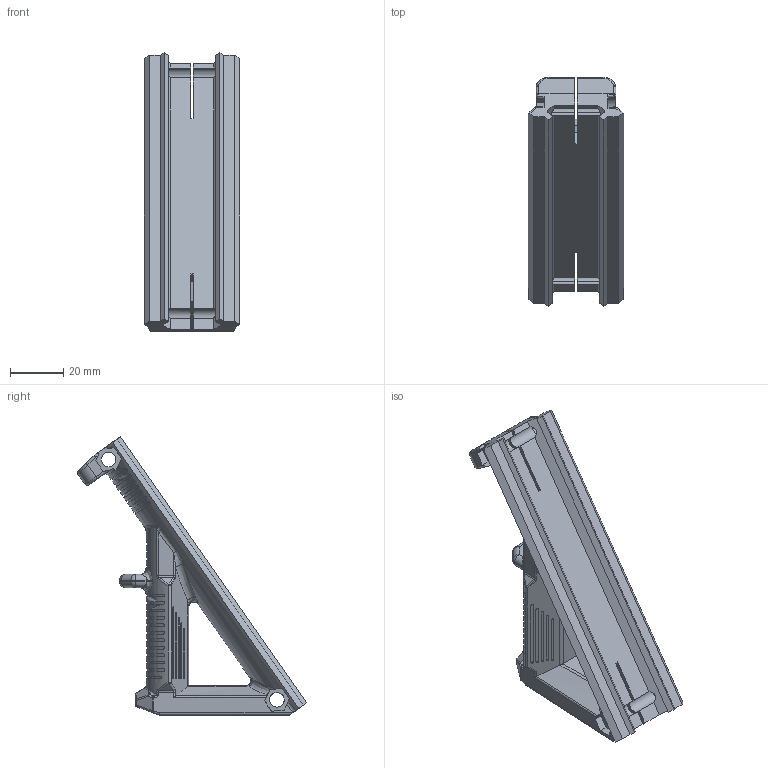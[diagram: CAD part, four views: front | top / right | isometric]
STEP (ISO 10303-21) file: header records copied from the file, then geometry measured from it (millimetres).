
FILE_DESCRIPTION (( 'STEP AP214' ), '1' );
FILE_NAME ('Magpul AFG.STEP', '2015-04-02T08:10:22', ( 'WarFairy' ), ( '' ), 'SwSTEP 2.0', 'SolidWorks 2013', '' );
FILE_SCHEMA (( 'AUTOMOTIVE_DESIGN' ));
Length unit declared in the file: millimetre
Products named in the file (1): Magpul AFG
Bounding box: 36.02 x 86.02 x 104.5 mm (x, y, z)
Volume: 56053.1 mm3; surface area: 21771.6 mm2
Topology: 1 solids, 1 shells, 590 faces, 1632 edges, 1038 vertices
Faces by surface type: cylinder 260, plane 202, bspline 84, sphere 32, torus 12
Entity records: 22299 total; most frequent: CARTESIAN_POINT 8045, ORIENTED_EDGE 3244, DIRECTION 2725, EDGE_CURVE 1622, VERTEX_POINT 1036, AXIS2_PLACEMENT_3D 1006, VECTOR 713, LINE 713
